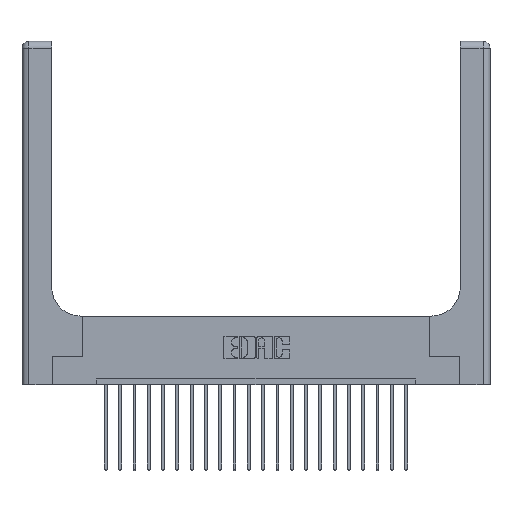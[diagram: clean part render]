
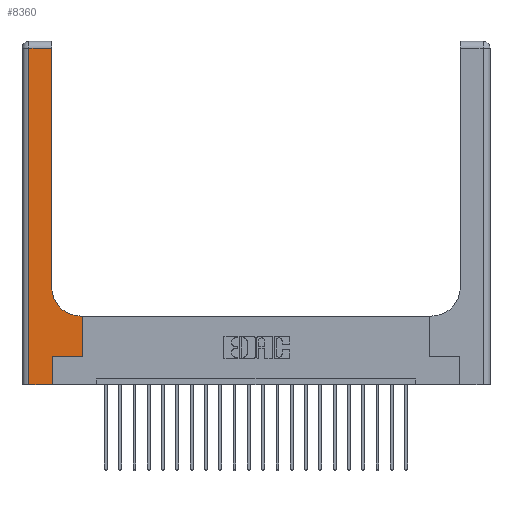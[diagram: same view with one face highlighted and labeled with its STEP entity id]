
A CAD part, top view. The second image highlights one B-rep face of the part: STEP entity #8360.
In plain terms, the highlighted planar face has unit normal (0, 0, 1).
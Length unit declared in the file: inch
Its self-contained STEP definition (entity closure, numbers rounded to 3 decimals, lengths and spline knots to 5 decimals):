
#386 = EDGE_CURVE ( 'NONE', #11522, #14468, #14168, .T. ) ;
#1188 = CARTESIAN_POINT ( 'NONE',  ( 0., 2.94, 0.37 ) ) ;
#1205 = ORIENTED_EDGE ( 'NONE', *, *, #1540, .T. ) ;
#1359 = VERTEX_POINT ( 'NONE', #12761 ) ;
#1510 = VECTOR ( 'NONE', #19663, 39.37008 ) ;
#1540 = EDGE_CURVE ( 'NONE', #11146, #11522, #13407, .T. ) ;
#1746 = CARTESIAN_POINT ( 'NONE',  ( 0.26, 0.6, 0.37 ) ) ;
#2390 = VERTEX_POINT ( 'NONE', #3143 ) ;
#2954 = VERTEX_POINT ( 'NONE', #20473 ) ;
#3143 = CARTESIAN_POINT ( 'NONE',  ( 0.265, 0.25, 0.37 ) ) ;
#3284 = ORIENTED_EDGE ( 'NONE', *, *, #4813, .T. ) ;
#3736 = AXIS2_PLACEMENT_3D ( 'NONE', #8412, #7196, #12078 ) ;
#4171 = ORIENTED_EDGE ( 'NONE', *, *, #10754, .T. ) ;
#4813 = EDGE_CURVE ( 'NONE', #1359, #12596, #5946, .T. ) ;
#4845 = VECTOR ( 'NONE', #7869, 39.37008 ) ;
#5176 = FACE_OUTER_BOUND ( 'NONE', #14909, .T. ) ;
#5946 = LINE ( 'NONE', #12635, #1510 ) ;
#5999 = DIRECTION ( 'NONE',  ( 1., 0., 0. ) ) ;
#6130 = CARTESIAN_POINT ( 'NONE',  ( 0.51, 0.85, 0.37 ) ) ;
#6145 = ORIENTED_EDGE ( 'NONE', *, *, #18557, .T. ) ;
#6185 = EDGE_CURVE ( 'NONE', #14468, #6795, #14146, .T. ) ;
#6289 = LINE ( 'NONE', #11529, #4845 ) ;
#6795 = VERTEX_POINT ( 'NONE', #8324 ) ;
#7072 = PLANE ( 'NONE',  #3736 ) ;
#7122 = EDGE_CURVE ( 'NONE', #11546, #2390, #21326, .T. ) ;
#7196 = DIRECTION ( 'NONE',  ( 0., 0., -1. ) ) ;
#7869 = DIRECTION ( 'NONE',  ( 1., 0., 0. ) ) ;
#8058 = LINE ( 'NONE', #11512, #13529 ) ;
#8324 = CARTESIAN_POINT ( 'NONE',  ( 0.26, 2.94, 0.37 ) ) ;
#8360 = ADVANCED_FACE ( 'NONE', ( #5176 ), #7072, .F. ) ;
#8412 = CARTESIAN_POINT ( 'NONE',  ( 0., 3., 0.37 ) ) ;
#8598 = ORIENTED_EDGE ( 'NONE', *, *, #7122, .T. ) ;
#8691 = VECTOR ( 'NONE', #18764, 39.37008 ) ;
#9619 = ORIENTED_EDGE ( 'NONE', *, *, #15699, .T. ) ;
#10404 = ORIENTED_EDGE ( 'NONE', *, *, #386, .T. ) ;
#10754 = EDGE_CURVE ( 'NONE', #2390, #2954, #6289, .T. ) ;
#11146 = VERTEX_POINT ( 'NONE', #13169 ) ;
#11192 = VECTOR ( 'NONE', #21265, 39.37008 ) ;
#11198 = CARTESIAN_POINT ( 'NONE',  ( 0.265, 0., 0.37 ) ) ;
#11403 = CARTESIAN_POINT ( 'NONE',  ( 0.06, 0., 0.37 ) ) ;
#11512 = CARTESIAN_POINT ( 'NONE',  ( 0.528, 0.25, 0.37 ) ) ;
#11522 = VERTEX_POINT ( 'NONE', #17272 ) ;
#11529 = CARTESIAN_POINT ( 'NONE',  ( 0.265, 0.25, 0.37 ) ) ;
#11546 = VERTEX_POINT ( 'NONE', #14286 ) ;
#11622 = LINE ( 'NONE', #1188, #17421 ) ;
#12078 = DIRECTION ( 'NONE',  ( -1., 0., 0. ) ) ;
#12485 = CARTESIAN_POINT ( 'NONE',  ( 0.26, 3., 0.37 ) ) ;
#12546 = ORIENTED_EDGE ( 'NONE', *, *, #17288, .T. ) ;
#12596 = VERTEX_POINT ( 'NONE', #11403 ) ;
#12635 = CARTESIAN_POINT ( 'NONE',  ( 0.06, 3., 0.37 ) ) ;
#12712 = DIRECTION ( 'NONE',  ( 1., 0., 0. ) ) ;
#12761 = CARTESIAN_POINT ( 'NONE',  ( 0.06, 2.94, 0.37 ) ) ;
#12877 = ORIENTED_EDGE ( 'NONE', *, *, #6185, .T. ) ;
#12915 = CARTESIAN_POINT ( 'NONE',  ( 0., 0., 0.37 ) ) ;
#12932 = DIRECTION ( 'NONE',  ( 0., 0., -1. ) ) ;
#13169 = CARTESIAN_POINT ( 'NONE',  ( 0.528, 0.6, 0.37 ) ) ;
#13407 = LINE ( 'NONE', #1746, #8691 ) ;
#13529 = VECTOR ( 'NONE', #16408, 39.37008 ) ;
#14146 = LINE ( 'NONE', #12485, #11192 ) ;
#14168 = CIRCLE ( 'NONE', #21289, 0.25 ) ;
#14286 = CARTESIAN_POINT ( 'NONE',  ( 0.265, 0., 0.37 ) ) ;
#14468 = VERTEX_POINT ( 'NONE', #16479 ) ;
#14909 = EDGE_LOOP ( 'NONE', ( #12877, #6145, #3284, #9619, #8598, #4171, #12546, #1205, #10404 ) ) ;
#14960 = DIRECTION ( 'NONE',  ( -1., 0., 0. ) ) ;
#15252 = VECTOR ( 'NONE', #5999, 39.37008 ) ;
#15699 = EDGE_CURVE ( 'NONE', #12596, #11546, #19382, .T. ) ;
#16408 = DIRECTION ( 'NONE',  ( 0., 1., 0. ) ) ;
#16479 = CARTESIAN_POINT ( 'NONE',  ( 0.26, 0.85, 0.37 ) ) ;
#17272 = CARTESIAN_POINT ( 'NONE',  ( 0.51, 0.6, 0.37 ) ) ;
#17288 = EDGE_CURVE ( 'NONE', #2954, #11146, #8058, .T. ) ;
#17421 = VECTOR ( 'NONE', #14960, 39.37008 ) ;
#17974 = DIRECTION ( 'NONE',  ( 0., 1., 0. ) ) ;
#18557 = EDGE_CURVE ( 'NONE', #6795, #1359, #11622, .T. ) ;
#18764 = DIRECTION ( 'NONE',  ( -1., 0., 0. ) ) ;
#19382 = LINE ( 'NONE', #12915, #15252 ) ;
#19414 = VECTOR ( 'NONE', #17974, 39.37008 ) ;
#19663 = DIRECTION ( 'NONE',  ( 0., -1., 0. ) ) ;
#20473 = CARTESIAN_POINT ( 'NONE',  ( 0.528, 0.25, 0.37 ) ) ;
#21265 = DIRECTION ( 'NONE',  ( 0., 1., 0. ) ) ;
#21289 = AXIS2_PLACEMENT_3D ( 'NONE', #6130, #12932, #12712 ) ;
#21326 = LINE ( 'NONE', #11198, #19414 ) ;
